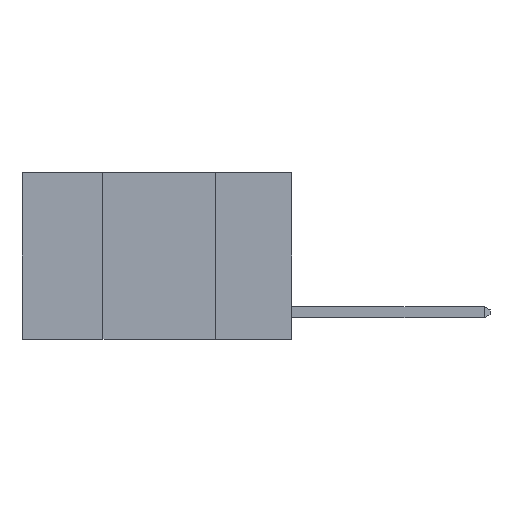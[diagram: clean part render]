
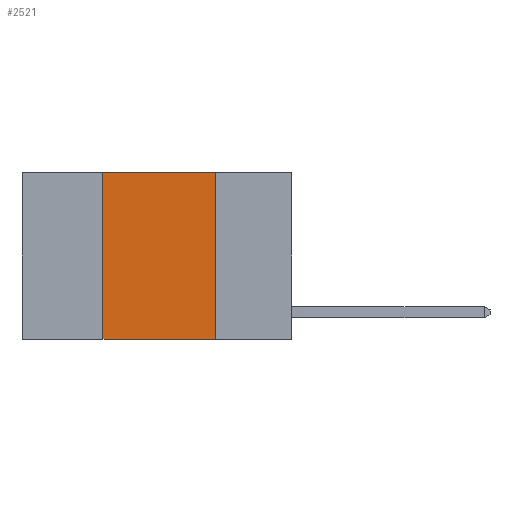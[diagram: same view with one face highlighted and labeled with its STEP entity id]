
A CAD part, left-side view. The second image highlights one B-rep face of the part: STEP entity #2521.
In plain terms, the highlighted planar face has unit normal (-1, 0, 0).
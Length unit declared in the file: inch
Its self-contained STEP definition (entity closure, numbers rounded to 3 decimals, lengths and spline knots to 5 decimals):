
#705 = CARTESIAN_POINT ( 'NONE',  ( 0., 0.6, 0. ) ) ;
#1745 = VECTOR ( 'NONE', #5399, 39.37008 ) ;
#1843 = VECTOR ( 'NONE', #10056, 39.37008 ) ;
#2044 = LINE ( 'NONE', #6330, #1745 ) ;
#2077 = EDGE_CURVE ( 'NONE', #6373, #2695, #4355, .T. ) ;
#2257 = CARTESIAN_POINT ( 'NONE',  ( 0., 0.17, -0.37 ) ) ;
#2340 = ORIENTED_EDGE ( 'NONE', *, *, #8951, .F. ) ;
#2468 = CARTESIAN_POINT ( 'NONE',  ( 0., 0.42, -0.37 ) ) ;
#2520 = ORIENTED_EDGE ( 'NONE', *, *, #2713, .F. ) ;
#2521 = ADVANCED_FACE ( 'NONE', ( #6207 ), #3135, .F. ) ;
#2601 = VECTOR ( 'NONE', #8420, 39.37008 ) ;
#2695 = VERTEX_POINT ( 'NONE', #2257 ) ;
#2713 = EDGE_CURVE ( 'NONE', #6373, #4762, #10962, .T. ) ;
#2952 = CARTESIAN_POINT ( 'NONE',  ( 0., 0.6, 0. ) ) ;
#3135 = PLANE ( 'NONE',  #4258 ) ;
#3950 = DIRECTION ( 'NONE',  ( 1., 0., 0. ) ) ;
#4160 = CARTESIAN_POINT ( 'NONE',  ( 0., 0.42, 0. ) ) ;
#4164 = ORIENTED_EDGE ( 'NONE', *, *, #4597, .F. ) ;
#4258 = AXIS2_PLACEMENT_3D ( 'NONE', #705, #3950, #4742 ) ;
#4355 = LINE ( 'NONE', #6762, #1843 ) ;
#4597 = EDGE_CURVE ( 'NONE', #8401, #2695, #2044, .T. ) ;
#4742 = DIRECTION ( 'NONE',  ( 0., 0., -1. ) ) ;
#4761 = CARTESIAN_POINT ( 'NONE',  ( 0., 0.42, 0. ) ) ;
#4762 = VERTEX_POINT ( 'NONE', #4761 ) ;
#5399 = DIRECTION ( 'NONE',  ( 0., 0., -1. ) ) ;
#6207 = FACE_OUTER_BOUND ( 'NONE', #11256, .T. ) ;
#6330 = CARTESIAN_POINT ( 'NONE',  ( 0., 0.17, 0. ) ) ;
#6373 = VERTEX_POINT ( 'NONE', #2468 ) ;
#6762 = CARTESIAN_POINT ( 'NONE',  ( 0., 0.6, -0.37 ) ) ;
#7775 = LINE ( 'NONE', #2952, #2601 ) ;
#8323 = CARTESIAN_POINT ( 'NONE',  ( 0., 0.17, 0. ) ) ;
#8401 = VERTEX_POINT ( 'NONE', #8323 ) ;
#8420 = DIRECTION ( 'NONE',  ( 0., -1., 0. ) ) ;
#8706 = VECTOR ( 'NONE', #9975, 39.37008 ) ;
#8951 = EDGE_CURVE ( 'NONE', #4762, #8401, #7775, .T. ) ;
#9975 = DIRECTION ( 'NONE',  ( 0., 0., 1. ) ) ;
#10056 = DIRECTION ( 'NONE',  ( 0., -1., 0. ) ) ;
#10404 = ORIENTED_EDGE ( 'NONE', *, *, #2077, .T. ) ;
#10962 = LINE ( 'NONE', #4160, #8706 ) ;
#11256 = EDGE_LOOP ( 'NONE', ( #4164, #2340, #2520, #10404 ) ) ;
